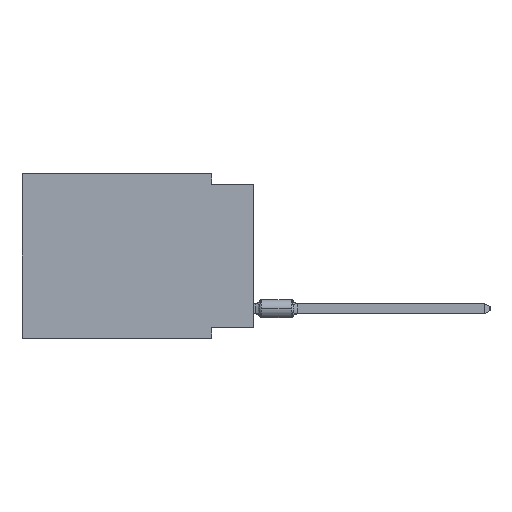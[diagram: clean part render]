
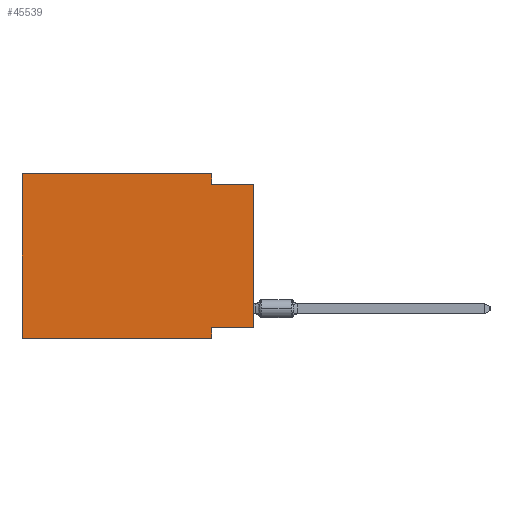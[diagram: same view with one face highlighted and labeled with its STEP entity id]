
A CAD part, left-side view. The second image highlights one B-rep face of the part: STEP entity #45539.
In plain terms, the highlighted planar face has unit normal (-1, 0, 0).
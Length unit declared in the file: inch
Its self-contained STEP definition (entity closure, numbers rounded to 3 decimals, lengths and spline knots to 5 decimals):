
#101 = CARTESIAN_POINT ( 'NONE',  ( 0., 0.55, 0. ) ) ;
#468 = VECTOR ( 'NONE', #32501, 39.37008 ) ;
#673 = CARTESIAN_POINT ( 'NONE',  ( 0., 0.55, -0.39 ) ) ;
#1089 = EDGE_CURVE ( 'NONE', #7417, #41491, #11370, .T. ) ;
#1417 = CARTESIAN_POINT ( 'NONE',  ( 0., 0.55, 0. ) ) ;
#1642 = VECTOR ( 'NONE', #3146, 39.37008 ) ;
#3146 = DIRECTION ( 'NONE',  ( 0., -1., 0. ) ) ;
#3792 = CARTESIAN_POINT ( 'NONE',  ( 0., 0.1, -0.39 ) ) ;
#3794 = CARTESIAN_POINT ( 'NONE',  ( 0., 0.1, -0.025 ) ) ;
#4132 = CARTESIAN_POINT ( 'NONE',  ( 0., 0., -0.025 ) ) ;
#4333 = ORIENTED_EDGE ( 'NONE', *, *, #31408, .F. ) ;
#4943 = VECTOR ( 'NONE', #22219, 39.37008 ) ;
#7417 = VERTEX_POINT ( 'NONE', #31463 ) ;
#7688 = FACE_OUTER_BOUND ( 'NONE', #26680, .T. ) ;
#8619 = EDGE_CURVE ( 'NONE', #27138, #19721, #31247, .T. ) ;
#8716 = VECTOR ( 'NONE', #33696, 39.37008 ) ;
#9458 = VERTEX_POINT ( 'NONE', #4132 ) ;
#9882 = CARTESIAN_POINT ( 'NONE',  ( 0., 0.1, -0.365 ) ) ;
#10129 = LINE ( 'NONE', #38074, #8716 ) ;
#11370 = LINE ( 'NONE', #12072, #4943 ) ;
#11622 = DIRECTION ( 'NONE',  ( 0., 0., -1. ) ) ;
#11892 = ORIENTED_EDGE ( 'NONE', *, *, #28403, .T. ) ;
#11947 = CARTESIAN_POINT ( 'NONE',  ( 0., 0.1, 0. ) ) ;
#12072 = CARTESIAN_POINT ( 'NONE',  ( 0., 0.55, 0. ) ) ;
#13025 = VERTEX_POINT ( 'NONE', #16025 ) ;
#14753 = EDGE_CURVE ( 'NONE', #13025, #9458, #25340, .T. ) ;
#15008 = ORIENTED_EDGE ( 'NONE', *, *, #1089, .F. ) ;
#15228 = VECTOR ( 'NONE', #36262, 39.37008 ) ;
#16025 = CARTESIAN_POINT ( 'NONE',  ( 0., 0., -0.365 ) ) ;
#16676 = ORIENTED_EDGE ( 'NONE', *, *, #29347, .F. ) ;
#17433 = ORIENTED_EDGE ( 'NONE', *, *, #32743, .F. ) ;
#18002 = VERTEX_POINT ( 'NONE', #11947 ) ;
#18548 = DIRECTION ( 'NONE',  ( 1., 0., 0. ) ) ;
#18895 = VECTOR ( 'NONE', #23857, 39.37008 ) ;
#18961 = VECTOR ( 'NONE', #28802, 39.37008 ) ;
#19721 = VERTEX_POINT ( 'NONE', #37774 ) ;
#21102 = LINE ( 'NONE', #34974, #1642 ) ;
#22219 = DIRECTION ( 'NONE',  ( 0., 0., 1. ) ) ;
#23020 = LINE ( 'NONE', #43615, #18895 ) ;
#23857 = DIRECTION ( 'NONE',  ( 0., 0., -1. ) ) ;
#25164 = VERTEX_POINT ( 'NONE', #3794 ) ;
#25340 = LINE ( 'NONE', #39439, #468 ) ;
#26466 = VECTOR ( 'NONE', #41900, 39.37008 ) ;
#26680 = EDGE_LOOP ( 'NONE', ( #38985, #4333, #36331, #17433, #15008, #11892, #35375, #16676 ) ) ;
#27138 = VERTEX_POINT ( 'NONE', #9882 ) ;
#27275 = EDGE_CURVE ( 'NONE', #18002, #25164, #23020, .T. ) ;
#28336 = LINE ( 'NONE', #673, #18961 ) ;
#28403 = EDGE_CURVE ( 'NONE', #7417, #19721, #28336, .T. ) ;
#28802 = DIRECTION ( 'NONE',  ( 0., -1., 0. ) ) ;
#28871 = CARTESIAN_POINT ( 'NONE',  ( 0., 0., -0.365 ) ) ;
#29347 = EDGE_CURVE ( 'NONE', #13025, #27138, #39746, .T. ) ;
#31247 = LINE ( 'NONE', #3792, #26466 ) ;
#31408 = EDGE_CURVE ( 'NONE', #25164, #9458, #10129, .T. ) ;
#31463 = CARTESIAN_POINT ( 'NONE',  ( 0., 0.55, -0.39 ) ) ;
#32501 = DIRECTION ( 'NONE',  ( 0., 0., 1. ) ) ;
#32743 = EDGE_CURVE ( 'NONE', #41491, #18002, #21102, .T. ) ;
#33696 = DIRECTION ( 'NONE',  ( 0., -1., 0. ) ) ;
#34974 = CARTESIAN_POINT ( 'NONE',  ( 0., 0.55, 0. ) ) ;
#35375 = ORIENTED_EDGE ( 'NONE', *, *, #8619, .F. ) ;
#36262 = DIRECTION ( 'NONE',  ( 0., 1., 0. ) ) ;
#36331 = ORIENTED_EDGE ( 'NONE', *, *, #27275, .F. ) ;
#37774 = CARTESIAN_POINT ( 'NONE',  ( 0., 0.1, -0.39 ) ) ;
#38074 = CARTESIAN_POINT ( 'NONE',  ( 0., 0., -0.025 ) ) ;
#38421 = AXIS2_PLACEMENT_3D ( 'NONE', #101, #18548, #11622 ) ;
#38985 = ORIENTED_EDGE ( 'NONE', *, *, #14753, .T. ) ;
#39439 = CARTESIAN_POINT ( 'NONE',  ( 0., 0., 0. ) ) ;
#39558 = PLANE ( 'NONE',  #38421 ) ;
#39746 = LINE ( 'NONE', #28871, #15228 ) ;
#41491 = VERTEX_POINT ( 'NONE', #1417 ) ;
#41900 = DIRECTION ( 'NONE',  ( 0., 0., -1. ) ) ;
#43615 = CARTESIAN_POINT ( 'NONE',  ( 0., 0.1, 0. ) ) ;
#45539 = ADVANCED_FACE ( 'NONE', ( #7688 ), #39558, .F. ) ;
